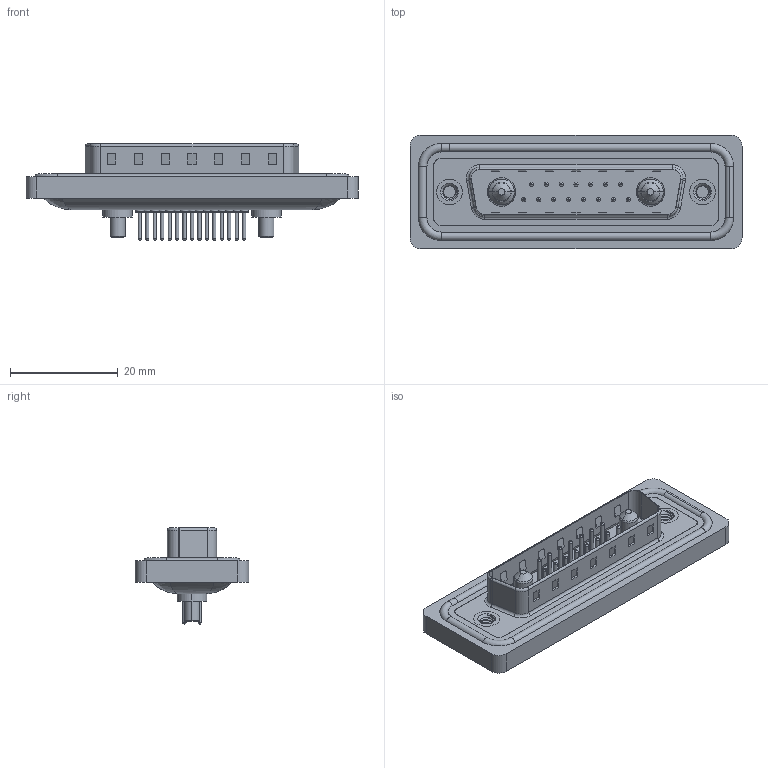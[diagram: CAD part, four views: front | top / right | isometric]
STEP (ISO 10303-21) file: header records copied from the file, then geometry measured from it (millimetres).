
FILE_DESCRIPTION (( 'STEP AP203' ), '1' );
FILE_NAME ('627W17W2224-2N2.STEP', '2024-03-19T20:31:09', ( '' ), ( '' ), 'SwSTEP 2.0', 'SolidWorks 2023', '' );
FILE_SCHEMA (( 'CONFIG_CONTROL_DESIGN' ));
Length unit declared in the file: millimetre
Products named in the file (9): 627Combo Housing_17W2; 627W17W2224-2N2; 627Combo Threaded Rivet_2; 627Combo Shell Front_25 Contacts; 627Combo Waterproof Housing_25 Contacts; Power Pin_20A S; 627Combo Contact Row 2_24; 627Combo Contact Row 1_24; 627Combo Shell Rear_25 Contacts
Assembly tree (23 placements, depth 2):
  627W17W2224-2N2
    627Combo Housing_17W2
    627Combo Waterproof Housing_25 Contacts
    627Combo Shell Rear_25 Contacts
    627Combo Shell Front_25 Contacts
    627Combo Threaded Rivet_2  x2
    Power Pin_20A S  x2
    627Combo Contact Row 1_24  x7
    627Combo Contact Row 2_24  x8
Bounding box: 61.75 x 21.1 x 17.9 mm (x, y, z)
Volume: 7266.4 mm3; surface area: 11914 mm2
Topology: 26 solids, 26 shells, 1116 faces, 2499 edges, 1529 vertices
Faces by surface type: cylinder 436, plane 334, torus 308, cone 26, bspline 12
Entity records: 22914 total; most frequent: CARTESIAN_POINT 5249, DIRECTION 3652, ORIENTED_EDGE 3228, EDGE_CURVE 1614, AXIS2_PLACEMENT_3D 1419, VERTEX_POINT 1019, VECTOR 814, LINE 814
